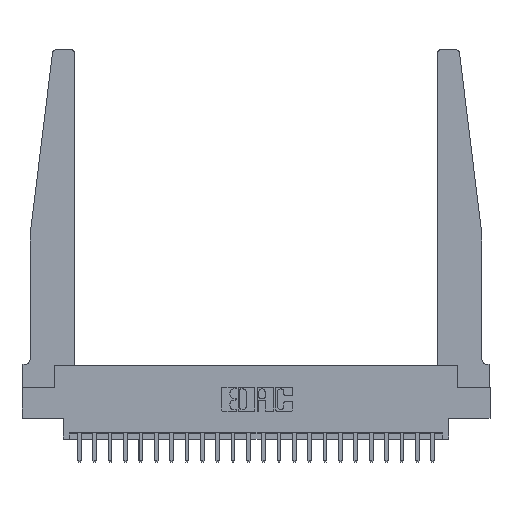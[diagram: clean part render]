
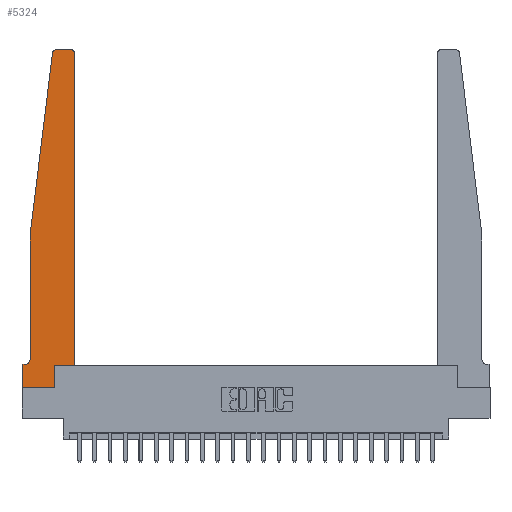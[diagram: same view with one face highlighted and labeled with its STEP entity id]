
A CAD part, top view. The second image highlights one B-rep face of the part: STEP entity #5324.
In plain terms, the highlighted planar face has unit normal (0, 0, 1).
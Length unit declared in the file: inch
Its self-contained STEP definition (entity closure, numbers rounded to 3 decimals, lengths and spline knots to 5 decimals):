
#27 = CARTESIAN_POINT ( 'NONE',  ( 0.2605, 0.18, 0.37 ) ) ;
#143 = CARTESIAN_POINT ( 'NONE',  ( 0.065, 1.25, 0.37 ) ) ;
#178 = DIRECTION ( 'NONE',  ( 1., 0., 0. ) ) ;
#414 = CIRCLE ( 'NONE', #17532, 0.03 ) ;
#991 = VECTOR ( 'NONE', #7710, 39.37008 ) ;
#1110 = DIRECTION ( 'NONE',  ( 0., -1., 0. ) ) ;
#1135 = CARTESIAN_POINT ( 'NONE',  ( 0.015, 0.1875, 0.37 ) ) ;
#1267 = EDGE_LOOP ( 'NONE', ( #10264, #4319, #18596, #16335, #11995, #20028, #5284, #17528, #14831, #6850, #3720, #21066 ) ) ;
#1314 = CARTESIAN_POINT ( 'NONE',  ( 0.425, 2.72, 0.37 ) ) ;
#2340 = EDGE_CURVE ( 'NONE', #23424, #15692, #13184, .T. ) ;
#2431 = EDGE_CURVE ( 'NONE', #15692, #7534, #4249, .T. ) ;
#2726 = VECTOR ( 'NONE', #12745, 39.37008 ) ;
#2830 = VECTOR ( 'NONE', #17849, 39.37008 ) ;
#2990 = CARTESIAN_POINT ( 'NONE',  ( 0.065, 1.25, 0.37 ) ) ;
#3141 = LINE ( 'NONE', #4929, #22484 ) ;
#3449 = EDGE_CURVE ( 'NONE', #8090, #22206, #414, .T. ) ;
#3720 = ORIENTED_EDGE ( 'NONE', *, *, #2431, .T. ) ;
#3809 = CARTESIAN_POINT ( 'NONE',  ( 0.2605, 0.18, 0.37 ) ) ;
#3995 = DIRECTION ( 'NONE',  ( 0., 0., 1. ) ) ;
#4005 = CARTESIAN_POINT ( 'NONE',  ( 0.015, 0.2375, 0.37 ) ) ;
#4229 = CARTESIAN_POINT ( 'NONE',  ( 0.395, 2.72, 0.37 ) ) ;
#4249 = LINE ( 'NONE', #16640, #991 ) ;
#4283 = LINE ( 'NONE', #7383, #7342 ) ;
#4319 = ORIENTED_EDGE ( 'NONE', *, *, #3449, .T. ) ;
#4863 = VERTEX_POINT ( 'NONE', #20494 ) ;
#4929 = CARTESIAN_POINT ( 'NONE',  ( 0., 0., 0.37 ) ) ;
#4990 = CARTESIAN_POINT ( 'NONE',  ( 0.065, 1.25, 0.37 ) ) ;
#5284 = ORIENTED_EDGE ( 'NONE', *, *, #17862, .T. ) ;
#5324 = ADVANCED_FACE ( 'NONE', ( #15331 ), #20687, .T. ) ;
#6314 = DIRECTION ( 'NONE',  ( 1., 0., 0. ) ) ;
#6382 = DIRECTION ( 'NONE',  ( 0., 0., 1. ) ) ;
#6850 = ORIENTED_EDGE ( 'NONE', *, *, #2340, .T. ) ;
#6909 = VECTOR ( 'NONE', #8476, 39.37008 ) ;
#7009 = LINE ( 'NONE', #4990, #2830 ) ;
#7252 = DIRECTION ( 'NONE',  ( -1., 0., 0. ) ) ;
#7342 = VECTOR ( 'NONE', #11309, 39.37008 ) ;
#7383 = CARTESIAN_POINT ( 'NONE',  ( 0.065, 0.1875, 0.37 ) ) ;
#7534 = VERTEX_POINT ( 'NONE', #1314 ) ;
#7710 = DIRECTION ( 'NONE',  ( 0., 1., 0. ) ) ;
#8090 = VERTEX_POINT ( 'NONE', #8914 ) ;
#8476 = DIRECTION ( 'NONE',  ( 0., -1., 0. ) ) ;
#8810 = CIRCLE ( 'NONE', #20225, 0.05 ) ;
#8914 = CARTESIAN_POINT ( 'NONE',  ( 0.27653, 2.75, 0.37 ) ) ;
#9382 = DIRECTION ( 'NONE',  ( 1., 0., 0. ) ) ;
#9483 = DIRECTION ( 'NONE',  ( -1., 0., 0. ) ) ;
#9495 = DIRECTION ( 'NONE',  ( 1., 0., 0. ) ) ;
#9614 = CARTESIAN_POINT ( 'NONE',  ( 0., 0., 0.37 ) ) ;
#9777 = DIRECTION ( 'NONE',  ( 0., 0., 1. ) ) ;
#9821 = AXIS2_PLACEMENT_3D ( 'NONE', #22363, #6382, #9843 ) ;
#9843 = DIRECTION ( 'NONE',  ( 1., 0., 0. ) ) ;
#9870 = EDGE_CURVE ( 'NONE', #15660, #21967, #8810, .T. ) ;
#10264 = ORIENTED_EDGE ( 'NONE', *, *, #12658, .T. ) ;
#10530 = VECTOR ( 'NONE', #9382, 39.37008 ) ;
#10941 = AXIS2_PLACEMENT_3D ( 'NONE', #4229, #3995, #178 ) ;
#11309 = DIRECTION ( 'NONE',  ( -1., 0., 0. ) ) ;
#11995 = ORIENTED_EDGE ( 'NONE', *, *, #9870, .T. ) ;
#12658 = EDGE_CURVE ( 'NONE', #16084, #8090, #21671, .T. ) ;
#12745 = DIRECTION ( 'NONE',  ( 0., 1., 0. ) ) ;
#12919 = VECTOR ( 'NONE', #7252, 39.37008 ) ;
#13184 = LINE ( 'NONE', #15204, #16976 ) ;
#13574 = CIRCLE ( 'NONE', #10941, 0.03 ) ;
#13740 = CARTESIAN_POINT ( 'NONE',  ( 0., 0., 0.37 ) ) ;
#14831 = ORIENTED_EDGE ( 'NONE', *, *, #18804, .T. ) ;
#15204 = CARTESIAN_POINT ( 'NONE',  ( 0.425, 0.18, 0.37 ) ) ;
#15263 = CARTESIAN_POINT ( 'NONE',  ( 0.27653, 2.72, 0.37 ) ) ;
#15331 = FACE_OUTER_BOUND ( 'NONE', #1267, .T. ) ;
#15509 = VERTEX_POINT ( 'NONE', #143 ) ;
#15660 = VERTEX_POINT ( 'NONE', #21669 ) ;
#15692 = VERTEX_POINT ( 'NONE', #21787 ) ;
#15779 = EDGE_CURVE ( 'NONE', #16560, #19589, #20463, .T. ) ;
#16084 = VERTEX_POINT ( 'NONE', #23183 ) ;
#16318 = EDGE_CURVE ( 'NONE', #7534, #16084, #13574, .T. ) ;
#16335 = ORIENTED_EDGE ( 'NONE', *, *, #18247, .T. ) ;
#16560 = VERTEX_POINT ( 'NONE', #13740 ) ;
#16640 = CARTESIAN_POINT ( 'NONE',  ( 0.425, 0.18, 0.37 ) ) ;
#16976 = VECTOR ( 'NONE', #9495, 39.37008 ) ;
#17528 = ORIENTED_EDGE ( 'NONE', *, *, #15779, .T. ) ;
#17532 = AXIS2_PLACEMENT_3D ( 'NONE', #15263, #9777, #6314 ) ;
#17849 = DIRECTION ( 'NONE',  ( -0.122, -0.992, 0. ) ) ;
#17862 = EDGE_CURVE ( 'NONE', #4863, #16560, #3141, .T. ) ;
#18247 = EDGE_CURVE ( 'NONE', #15509, #15660, #20981, .T. ) ;
#18532 = DIRECTION ( 'NONE',  ( 0., 0., -1. ) ) ;
#18577 = LINE ( 'NONE', #3809, #2726 ) ;
#18596 = ORIENTED_EDGE ( 'NONE', *, *, #21615, .T. ) ;
#18804 = EDGE_CURVE ( 'NONE', #19589, #23424, #18577, .T. ) ;
#19589 = VERTEX_POINT ( 'NONE', #20513 ) ;
#19638 = CARTESIAN_POINT ( 'NONE',  ( 0.25, 2.75, 0.37 ) ) ;
#20028 = ORIENTED_EDGE ( 'NONE', *, *, #20095, .T. ) ;
#20095 = EDGE_CURVE ( 'NONE', #21967, #4863, #4283, .T. ) ;
#20225 = AXIS2_PLACEMENT_3D ( 'NONE', #4005, #18532, #9483 ) ;
#20315 = CARTESIAN_POINT ( 'NONE',  ( 0.24675, 2.72367, 0.37 ) ) ;
#20463 = LINE ( 'NONE', #9614, #10530 ) ;
#20494 = CARTESIAN_POINT ( 'NONE',  ( 0., 0.1875, 0.37 ) ) ;
#20513 = CARTESIAN_POINT ( 'NONE',  ( 0.2605, 0., 0.37 ) ) ;
#20687 = PLANE ( 'NONE',  #9821 ) ;
#20981 = LINE ( 'NONE', #2990, #6909 ) ;
#21066 = ORIENTED_EDGE ( 'NONE', *, *, #16318, .T. ) ;
#21615 = EDGE_CURVE ( 'NONE', #22206, #15509, #7009, .T. ) ;
#21669 = CARTESIAN_POINT ( 'NONE',  ( 0.065, 0.2375, 0.37 ) ) ;
#21671 = LINE ( 'NONE', #19638, #12919 ) ;
#21787 = CARTESIAN_POINT ( 'NONE',  ( 0.425, 0.18, 0.37 ) ) ;
#21967 = VERTEX_POINT ( 'NONE', #1135 ) ;
#22206 = VERTEX_POINT ( 'NONE', #20315 ) ;
#22363 = CARTESIAN_POINT ( 'NONE',  ( 0., 0.1875, 0.37 ) ) ;
#22484 = VECTOR ( 'NONE', #1110, 39.37008 ) ;
#23183 = CARTESIAN_POINT ( 'NONE',  ( 0.395, 2.75, 0.37 ) ) ;
#23424 = VERTEX_POINT ( 'NONE', #27 ) ;
